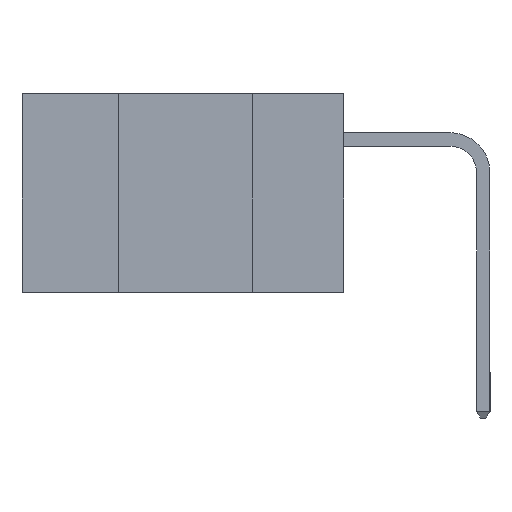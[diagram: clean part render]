
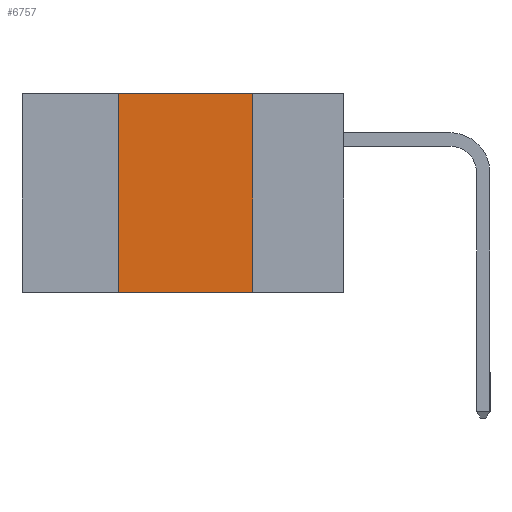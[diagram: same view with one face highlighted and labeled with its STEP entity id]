
A CAD part, left-side view. The second image highlights one B-rep face of the part: STEP entity #6757.
In plain terms, the highlighted planar face has unit normal (-1, 0, 0).
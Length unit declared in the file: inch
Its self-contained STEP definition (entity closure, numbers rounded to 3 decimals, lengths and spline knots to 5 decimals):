
#165 = DIRECTION ( 'NONE',  ( 0., 0., 1. ) ) ;
#192 = ORIENTED_EDGE ( 'NONE', *, *, #10940, .F. ) ;
#456 = VECTOR ( 'NONE', #165, 39.37008 ) ;
#516 = VECTOR ( 'NONE', #5675, 39.37008 ) ;
#894 = VERTEX_POINT ( 'NONE', #10167 ) ;
#1620 = LINE ( 'NONE', #7737, #6553 ) ;
#2018 = EDGE_CURVE ( 'NONE', #9825, #894, #8912, .T. ) ;
#2254 = LINE ( 'NONE', #5535, #456 ) ;
#2294 = CARTESIAN_POINT ( 'NONE',  ( 0., 0.17, -0.37 ) ) ;
#2341 = DIRECTION ( 'NONE',  ( 0., 0., -1. ) ) ;
#2662 = EDGE_LOOP ( 'NONE', ( #192, #4623, #4111, #13538 ) ) ;
#2977 = FACE_OUTER_BOUND ( 'NONE', #2662, .T. ) ;
#3586 = DIRECTION ( 'NONE',  ( 0., 0., -1. ) ) ;
#3620 = VERTEX_POINT ( 'NONE', #2294 ) ;
#3748 = EDGE_CURVE ( 'NONE', #6314, #3620, #1620, .T. ) ;
#4085 = CARTESIAN_POINT ( 'NONE',  ( 0., 0.42, 0. ) ) ;
#4111 = ORIENTED_EDGE ( 'NONE', *, *, #4555, .F. ) ;
#4555 = EDGE_CURVE ( 'NONE', #6314, #9825, #2254, .T. ) ;
#4623 = ORIENTED_EDGE ( 'NONE', *, *, #2018, .F. ) ;
#4821 = LINE ( 'NONE', #9873, #8938 ) ;
#5535 = CARTESIAN_POINT ( 'NONE',  ( 0., 0.42, 0. ) ) ;
#5675 = DIRECTION ( 'NONE',  ( 0., -1., 0. ) ) ;
#6268 = CARTESIAN_POINT ( 'NONE',  ( 0., 0.42, -0.37 ) ) ;
#6314 = VERTEX_POINT ( 'NONE', #6268 ) ;
#6540 = AXIS2_PLACEMENT_3D ( 'NONE', #11835, #12980, #2341 ) ;
#6553 = VECTOR ( 'NONE', #11901, 39.37008 ) ;
#6757 = ADVANCED_FACE ( 'NONE', ( #2977 ), #12930, .F. ) ;
#7737 = CARTESIAN_POINT ( 'NONE',  ( 0., 0.6, -0.37 ) ) ;
#8912 = LINE ( 'NONE', #12962, #516 ) ;
#8938 = VECTOR ( 'NONE', #3586, 39.37008 ) ;
#9825 = VERTEX_POINT ( 'NONE', #4085 ) ;
#9873 = CARTESIAN_POINT ( 'NONE',  ( 0., 0.17, 0. ) ) ;
#10167 = CARTESIAN_POINT ( 'NONE',  ( 0., 0.17, 0. ) ) ;
#10940 = EDGE_CURVE ( 'NONE', #894, #3620, #4821, .T. ) ;
#11835 = CARTESIAN_POINT ( 'NONE',  ( 0., 0.6, 0. ) ) ;
#11901 = DIRECTION ( 'NONE',  ( 0., -1., 0. ) ) ;
#12930 = PLANE ( 'NONE',  #6540 ) ;
#12962 = CARTESIAN_POINT ( 'NONE',  ( 0., 0.6, 0. ) ) ;
#12980 = DIRECTION ( 'NONE',  ( 1., 0., 0. ) ) ;
#13538 = ORIENTED_EDGE ( 'NONE', *, *, #3748, .T. ) ;
